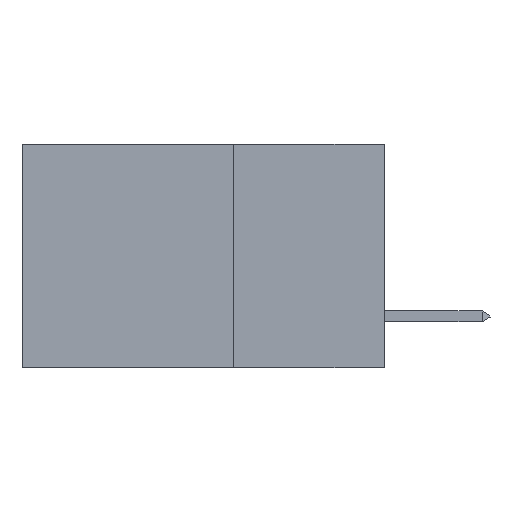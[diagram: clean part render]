
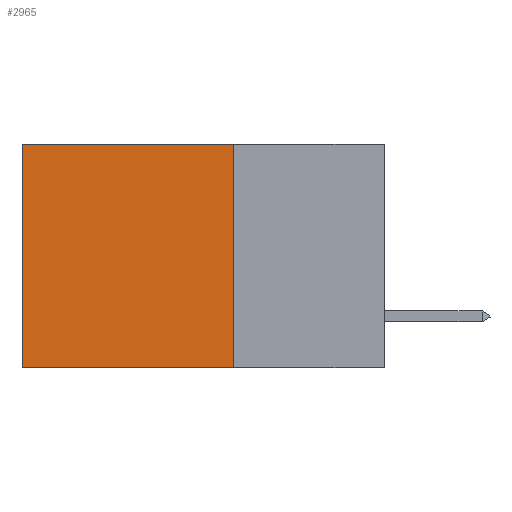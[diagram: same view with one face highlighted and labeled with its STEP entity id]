
A CAD part, left-side view. The second image highlights one B-rep face of the part: STEP entity #2965.
In plain terms, the highlighted planar face has unit normal (-1, 0, 0).
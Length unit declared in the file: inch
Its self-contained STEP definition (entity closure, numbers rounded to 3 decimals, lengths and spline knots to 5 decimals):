
#141 = VECTOR ( 'NONE', #19036, 39.37008 ) ;
#612 = CARTESIAN_POINT ( 'NONE',  ( 0.2875, 0.25, 0. ) ) ;
#1127 = VERTEX_POINT ( 'NONE', #8031 ) ;
#1188 = CARTESIAN_POINT ( 'NONE',  ( 0.2875, 0.6, 0. ) ) ;
#1852 = LINE ( 'NONE', #14571, #12194 ) ;
#2043 = ORIENTED_EDGE ( 'NONE', *, *, #9009, .F. ) ;
#2186 = ORIENTED_EDGE ( 'NONE', *, *, #7450, .F. ) ;
#2262 = DIRECTION ( 'NONE',  ( 0., 0., -1. ) ) ;
#2965 = ADVANCED_FACE ( 'NONE', ( #13120 ), #7316, .F. ) ;
#3446 = CARTESIAN_POINT ( 'NONE',  ( 0.2875, 0.25, -0.37 ) ) ;
#4456 = VECTOR ( 'NONE', #12476, 39.37008 ) ;
#5806 = CARTESIAN_POINT ( 'NONE',  ( 0.2875, 0.25, 0. ) ) ;
#7175 = CARTESIAN_POINT ( 'NONE',  ( 0.2875, 0.25, 0. ) ) ;
#7316 = PLANE ( 'NONE',  #8537 ) ;
#7450 = EDGE_CURVE ( 'NONE', #17496, #1127, #8089, .T. ) ;
#8031 = CARTESIAN_POINT ( 'NONE',  ( 0.2875, 0.25, -0.37 ) ) ;
#8089 = LINE ( 'NONE', #11140, #141 ) ;
#8537 = AXIS2_PLACEMENT_3D ( 'NONE', #7175, #10231, #18080 ) ;
#9009 = EDGE_CURVE ( 'NONE', #1127, #13179, #11319, .T. ) ;
#9420 = ORIENTED_EDGE ( 'NONE', *, *, #17260, .T. ) ;
#9699 = LINE ( 'NONE', #5806, #4456 ) ;
#9982 = VERTEX_POINT ( 'NONE', #1188 ) ;
#10231 = DIRECTION ( 'NONE',  ( 1., 0., 0. ) ) ;
#10544 = CARTESIAN_POINT ( 'NONE',  ( 0.2875, 0.6, -0.37 ) ) ;
#10962 = EDGE_CURVE ( 'NONE', #9982, #13179, #1852, .T. ) ;
#11140 = CARTESIAN_POINT ( 'NONE',  ( 0.2875, 0.25, 0. ) ) ;
#11319 = LINE ( 'NONE', #3446, #18807 ) ;
#12194 = VECTOR ( 'NONE', #2262, 39.37008 ) ;
#12476 = DIRECTION ( 'NONE',  ( 0., 1., 0. ) ) ;
#12810 = EDGE_LOOP ( 'NONE', ( #14504, #2043, #2186, #9420 ) ) ;
#13120 = FACE_OUTER_BOUND ( 'NONE', #12810, .T. ) ;
#13179 = VERTEX_POINT ( 'NONE', #10544 ) ;
#14079 = DIRECTION ( 'NONE',  ( 0., 1., 0. ) ) ;
#14504 = ORIENTED_EDGE ( 'NONE', *, *, #10962, .T. ) ;
#14571 = CARTESIAN_POINT ( 'NONE',  ( 0.2875, 0.6, 0. ) ) ;
#17260 = EDGE_CURVE ( 'NONE', #17496, #9982, #9699, .T. ) ;
#17496 = VERTEX_POINT ( 'NONE', #612 ) ;
#18080 = DIRECTION ( 'NONE',  ( 0., 0., -1. ) ) ;
#18807 = VECTOR ( 'NONE', #14079, 39.37008 ) ;
#19036 = DIRECTION ( 'NONE',  ( 0., 0., -1. ) ) ;
